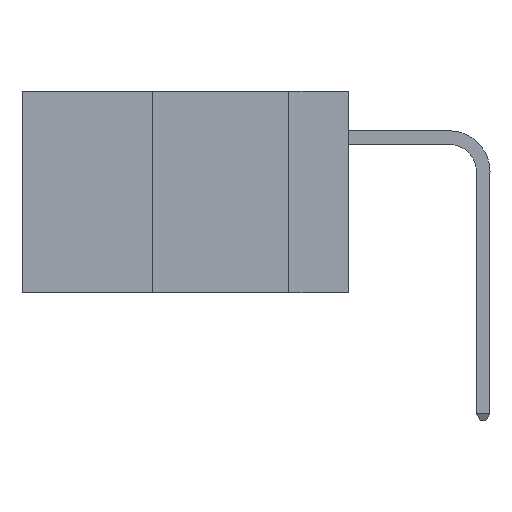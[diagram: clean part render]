
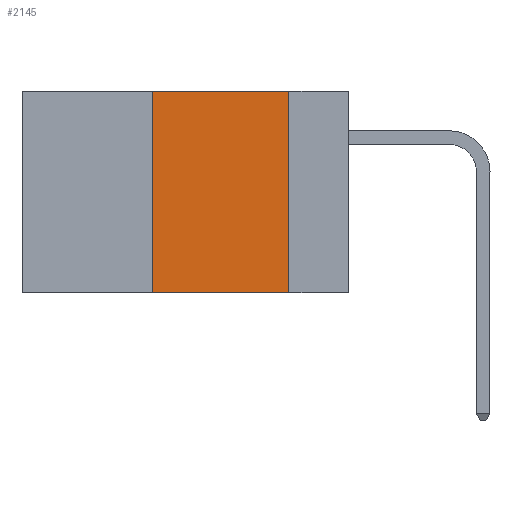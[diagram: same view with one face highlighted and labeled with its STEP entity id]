
A CAD part, left-side view. The second image highlights one B-rep face of the part: STEP entity #2145.
In plain terms, the highlighted planar face has unit normal (-1, 0, 0).
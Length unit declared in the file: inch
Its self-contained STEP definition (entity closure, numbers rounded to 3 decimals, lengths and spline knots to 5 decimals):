
#92 = VERTEX_POINT ( 'NONE', #8174 ) ;
#722 = VECTOR ( 'NONE', #15950, 39.37008 ) ;
#2145 = ADVANCED_FACE ( 'NONE', ( #16863 ), #13914, .F. ) ;
#2764 = DIRECTION ( 'NONE',  ( 0., -1., 0. ) ) ;
#3196 = VECTOR ( 'NONE', #5015, 39.37008 ) ;
#3380 = LINE ( 'NONE', #16584, #15434 ) ;
#3683 = CARTESIAN_POINT ( 'NONE',  ( 0., 0.11, 0. ) ) ;
#5015 = DIRECTION ( 'NONE',  ( 0., -1., 0. ) ) ;
#5814 = CARTESIAN_POINT ( 'NONE',  ( 0., 0.36, 0. ) ) ;
#6446 = VERTEX_POINT ( 'NONE', #21011 ) ;
#6560 = CARTESIAN_POINT ( 'NONE',  ( 0., 0.36, -0.37 ) ) ;
#6617 = ORIENTED_EDGE ( 'NONE', *, *, #6832, .F. ) ;
#6832 = EDGE_CURVE ( 'NONE', #6446, #92, #3380, .T. ) ;
#7020 = LINE ( 'NONE', #3683, #722 ) ;
#7647 = DIRECTION ( 'NONE',  ( 0., 0., 1. ) ) ;
#8174 = CARTESIAN_POINT ( 'NONE',  ( 0., 0.11, 0. ) ) ;
#8552 = CARTESIAN_POINT ( 'NONE',  ( 0., 0.6, 0. ) ) ;
#8712 = DIRECTION ( 'NONE',  ( 0., 0., -1. ) ) ;
#10001 = VERTEX_POINT ( 'NONE', #6560 ) ;
#11614 = ORIENTED_EDGE ( 'NONE', *, *, #20389, .F. ) ;
#13870 = CARTESIAN_POINT ( 'NONE',  ( 0., 0.6, -0.37 ) ) ;
#13914 = PLANE ( 'NONE',  #19861 ) ;
#15434 = VECTOR ( 'NONE', #2764, 39.37008 ) ;
#15658 = DIRECTION ( 'NONE',  ( 1., 0., 0. ) ) ;
#15950 = DIRECTION ( 'NONE',  ( 0., 0., -1. ) ) ;
#16366 = CARTESIAN_POINT ( 'NONE',  ( 0., 0.11, -0.37 ) ) ;
#16466 = VERTEX_POINT ( 'NONE', #16366 ) ;
#16584 = CARTESIAN_POINT ( 'NONE',  ( 0., 0.6, 0. ) ) ;
#16863 = FACE_OUTER_BOUND ( 'NONE', #19308, .T. ) ;
#17349 = VECTOR ( 'NONE', #7647, 39.37008 ) ;
#19308 = EDGE_LOOP ( 'NONE', ( #11614, #6617, #20393, #19510 ) ) ;
#19510 = ORIENTED_EDGE ( 'NONE', *, *, #20683, .T. ) ;
#19533 = LINE ( 'NONE', #13870, #3196 ) ;
#19861 = AXIS2_PLACEMENT_3D ( 'NONE', #8552, #15658, #8712 ) ;
#20389 = EDGE_CURVE ( 'NONE', #92, #16466, #7020, .T. ) ;
#20393 = ORIENTED_EDGE ( 'NONE', *, *, #20484, .F. ) ;
#20484 = EDGE_CURVE ( 'NONE', #10001, #6446, #21390, .T. ) ;
#20683 = EDGE_CURVE ( 'NONE', #10001, #16466, #19533, .T. ) ;
#21011 = CARTESIAN_POINT ( 'NONE',  ( 0., 0.36, 0. ) ) ;
#21390 = LINE ( 'NONE', #5814, #17349 ) ;
